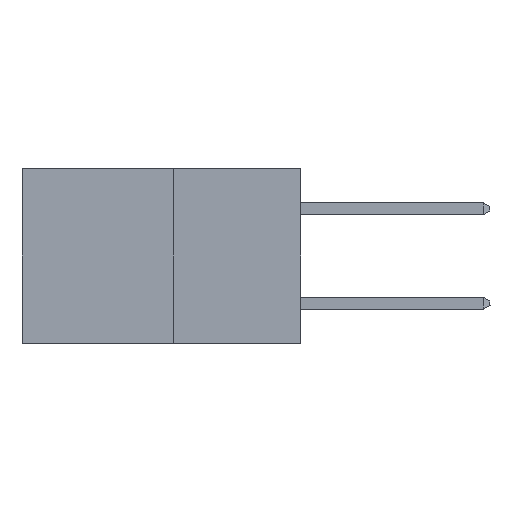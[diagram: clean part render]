
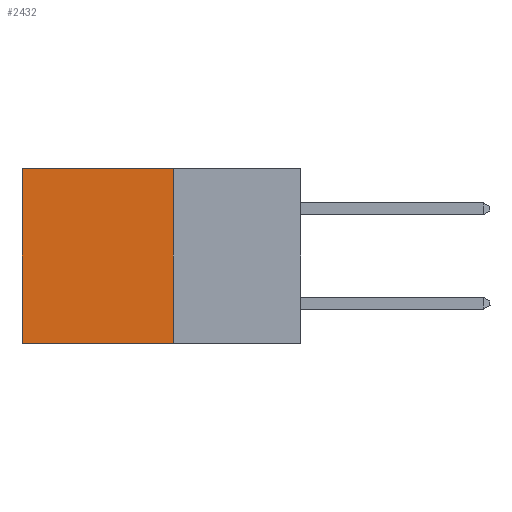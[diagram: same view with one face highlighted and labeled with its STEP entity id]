
A CAD part, left-side view. The second image highlights one B-rep face of the part: STEP entity #2432.
In plain terms, the highlighted planar face has unit normal (-1, 0, 0).
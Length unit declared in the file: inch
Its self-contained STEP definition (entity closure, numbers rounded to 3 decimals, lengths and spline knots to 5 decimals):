
#655 = VECTOR ( 'NONE', #5332, 39.37008 ) ;
#1472 = ORIENTED_EDGE ( 'NONE', *, *, #6317, .T. ) ;
#1530 = ORIENTED_EDGE ( 'NONE', *, *, #4040, .T. ) ;
#1844 = ORIENTED_EDGE ( 'NONE', *, *, #13126, .F. ) ;
#2432 = ADVANCED_FACE ( 'NONE', ( #11407 ), #6175, .F. ) ;
#2652 = CARTESIAN_POINT ( 'NONE',  ( 0.277, 0.27, -0.37 ) ) ;
#2688 = VECTOR ( 'NONE', #6425, 39.37008 ) ;
#2813 = CARTESIAN_POINT ( 'NONE',  ( 0.277, 0.59, 0. ) ) ;
#3288 = DIRECTION ( 'NONE',  ( 0., 0., -1. ) ) ;
#3361 = VERTEX_POINT ( 'NONE', #13076 ) ;
#3912 = LINE ( 'NONE', #6347, #655 ) ;
#4040 = EDGE_CURVE ( 'NONE', #11352, #9003, #8657, .T. ) ;
#4265 = VERTEX_POINT ( 'NONE', #6128 ) ;
#5332 = DIRECTION ( 'NONE',  ( 0., 1., 0. ) ) ;
#5643 = ORIENTED_EDGE ( 'NONE', *, *, #12020, .F. ) ;
#5698 = DIRECTION ( 'NONE',  ( 1., 0., 0. ) ) ;
#5918 = VECTOR ( 'NONE', #8980, 39.37008 ) ;
#6128 = CARTESIAN_POINT ( 'NONE',  ( 0.277, 0.59, -0.37 ) ) ;
#6175 = PLANE ( 'NONE',  #7912 ) ;
#6317 = EDGE_CURVE ( 'NONE', #9003, #4265, #10949, .T. ) ;
#6347 = CARTESIAN_POINT ( 'NONE',  ( 0.277, 0.27, -0.37 ) ) ;
#6425 = DIRECTION ( 'NONE',  ( 0., 0., -1. ) ) ;
#6462 = CARTESIAN_POINT ( 'NONE',  ( 0.277, 0.59, -0.37 ) ) ;
#6534 = CARTESIAN_POINT ( 'NONE',  ( 0.277, 0.27, -0.37 ) ) ;
#7912 = AXIS2_PLACEMENT_3D ( 'NONE', #2652, #5698, #12041 ) ;
#8657 = LINE ( 'NONE', #9091, #5918 ) ;
#8980 = DIRECTION ( 'NONE',  ( 0., 1., 0. ) ) ;
#9003 = VERTEX_POINT ( 'NONE', #2813 ) ;
#9091 = CARTESIAN_POINT ( 'NONE',  ( 0.277, 0.27, 0. ) ) ;
#10322 = LINE ( 'NONE', #6534, #13403 ) ;
#10949 = LINE ( 'NONE', #6462, #2688 ) ;
#11352 = VERTEX_POINT ( 'NONE', #13900 ) ;
#11407 = FACE_OUTER_BOUND ( 'NONE', #13349, .T. ) ;
#12020 = EDGE_CURVE ( 'NONE', #3361, #4265, #3912, .T. ) ;
#12041 = DIRECTION ( 'NONE',  ( 0., 0., -1. ) ) ;
#13076 = CARTESIAN_POINT ( 'NONE',  ( 0.277, 0.27, -0.37 ) ) ;
#13126 = EDGE_CURVE ( 'NONE', #11352, #3361, #10322, .T. ) ;
#13349 = EDGE_LOOP ( 'NONE', ( #1472, #5643, #1844, #1530 ) ) ;
#13403 = VECTOR ( 'NONE', #3288, 39.37008 ) ;
#13900 = CARTESIAN_POINT ( 'NONE',  ( 0.277, 0.27, 0. ) ) ;
